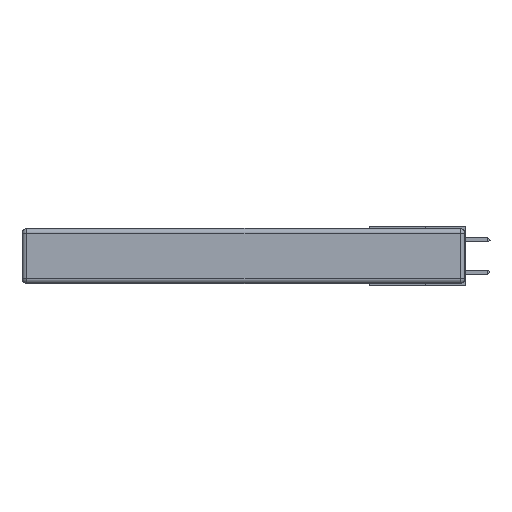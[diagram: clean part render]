
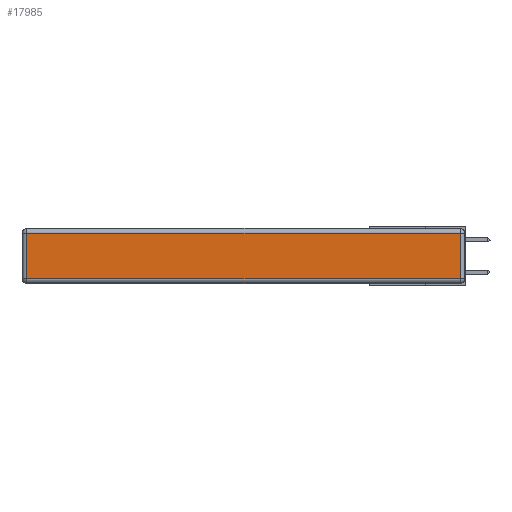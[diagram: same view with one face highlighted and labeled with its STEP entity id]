
A CAD part, left-side view. The second image highlights one B-rep face of the part: STEP entity #17985.
In plain terms, the highlighted planar face has unit normal (-1, 0, 0).
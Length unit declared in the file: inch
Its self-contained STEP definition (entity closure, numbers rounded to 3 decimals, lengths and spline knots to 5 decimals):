
#1057 = DIRECTION ( 'NONE',  ( -1., 0., 0. ) ) ;
#2284 = CARTESIAN_POINT ( 'NONE',  ( 0., 2.72, -0.03 ) ) ;
#2622 = CARTESIAN_POINT ( 'NONE',  ( 0., 2.75, -0.03 ) ) ;
#2677 = LINE ( 'NONE', #15140, #16349 ) ;
#3815 = VECTOR ( 'NONE', #15860, 39.37008 ) ;
#5691 = ORIENTED_EDGE ( 'NONE', *, *, #19010, .T. ) ;
#6391 = EDGE_CURVE ( 'NONE', #11767, #10144, #7772, .T. ) ;
#6924 = EDGE_CURVE ( 'NONE', #20888, #11767, #14584, .T. ) ;
#7772 = LINE ( 'NONE', #2622, #3815 ) ;
#7900 = ORIENTED_EDGE ( 'NONE', *, *, #6924, .T. ) ;
#9399 = CARTESIAN_POINT ( 'NONE',  ( 0., 0., -0.343 ) ) ;
#9602 = VECTOR ( 'NONE', #13637, 39.37008 ) ;
#10144 = VERTEX_POINT ( 'NONE', #2284 ) ;
#11143 = LINE ( 'NONE', #11295, #18781 ) ;
#11295 = CARTESIAN_POINT ( 'NONE',  ( 0., 2.72, -0.343 ) ) ;
#11767 = VERTEX_POINT ( 'NONE', #16661 ) ;
#12902 = DIRECTION ( 'NONE',  ( 0., 0., 1. ) ) ;
#12923 = ORIENTED_EDGE ( 'NONE', *, *, #6391, .T. ) ;
#13637 = DIRECTION ( 'NONE',  ( 0., 0., 1. ) ) ;
#14584 = LINE ( 'NONE', #18718, #9602 ) ;
#15140 = CARTESIAN_POINT ( 'NONE',  ( 0., 0., -0.313 ) ) ;
#15860 = DIRECTION ( 'NONE',  ( 0., 1., 0. ) ) ;
#16272 = VERTEX_POINT ( 'NONE', #21134 ) ;
#16349 = VECTOR ( 'NONE', #18760, 39.37008 ) ;
#16661 = CARTESIAN_POINT ( 'NONE',  ( 0., 0.03, -0.03 ) ) ;
#17214 = EDGE_LOOP ( 'NONE', ( #5691, #7900, #12923, #19820 ) ) ;
#17475 = EDGE_CURVE ( 'NONE', #10144, #16272, #11143, .T. ) ;
#17985 = ADVANCED_FACE ( 'NONE', ( #18766 ), #19590, .T. ) ;
#18046 = CARTESIAN_POINT ( 'NONE',  ( 0., 0.03, -0.313 ) ) ;
#18718 = CARTESIAN_POINT ( 'NONE',  ( 0., 0.03, -0.343 ) ) ;
#18760 = DIRECTION ( 'NONE',  ( 0., -1., 0. ) ) ;
#18766 = FACE_OUTER_BOUND ( 'NONE', #17214, .T. ) ;
#18781 = VECTOR ( 'NONE', #21578, 39.37008 ) ;
#19010 = EDGE_CURVE ( 'NONE', #16272, #20888, #2677, .T. ) ;
#19590 = PLANE ( 'NONE',  #20633 ) ;
#19820 = ORIENTED_EDGE ( 'NONE', *, *, #17475, .T. ) ;
#20633 = AXIS2_PLACEMENT_3D ( 'NONE', #9399, #1057, #12902 ) ;
#20888 = VERTEX_POINT ( 'NONE', #18046 ) ;
#21134 = CARTESIAN_POINT ( 'NONE',  ( 0., 2.72, -0.313 ) ) ;
#21578 = DIRECTION ( 'NONE',  ( 0., 0., -1. ) ) ;
